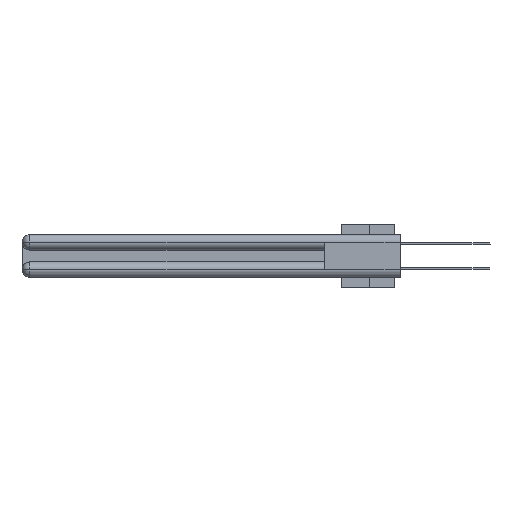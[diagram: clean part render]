
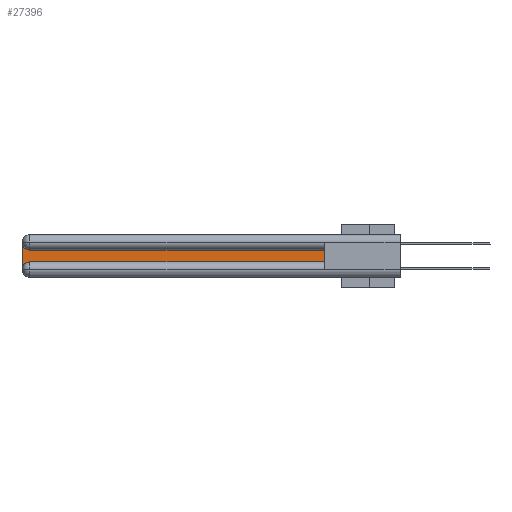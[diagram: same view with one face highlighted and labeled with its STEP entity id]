
A CAD part, left-side view. The second image highlights one B-rep face of the part: STEP entity #27396.
In plain terms, the highlighted planar face has unit normal (-1, 0, 0).
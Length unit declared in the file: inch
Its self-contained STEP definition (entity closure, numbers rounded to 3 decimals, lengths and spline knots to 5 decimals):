
#108 = VECTOR ( 'NONE', #23866, 39.37008 ) ;
#778 = CARTESIAN_POINT ( 'NONE',  ( 0.075, 3., -0.0625 ) ) ;
#1190 = CARTESIAN_POINT ( 'NONE',  ( 0.075, 2.94, -0.0625 ) ) ;
#3281 = CARTESIAN_POINT ( 'NONE',  ( 0.075, 0.6, -0.2175 ) ) ;
#3515 = LINE ( 'NONE', #32475, #12928 ) ;
#4697 = VERTEX_POINT ( 'NONE', #26727 ) ;
#5499 = AXIS2_PLACEMENT_3D ( 'NONE', #1190, #24079, #8109 ) ;
#5734 = VECTOR ( 'NONE', #16080, 39.37008 ) ;
#7492 = DIRECTION ( 'NONE',  ( 0., 0., -1. ) ) ;
#8109 = DIRECTION ( 'NONE',  ( 0., 0., -1. ) ) ;
#8886 = DIRECTION ( 'NONE',  ( 1., 0., 0. ) ) ;
#9432 = CARTESIAN_POINT ( 'NONE',  ( 0.075, 3., -0.2775 ) ) ;
#9581 = EDGE_LOOP ( 'NONE', ( #19163, #36787, #32205, #24450, #29224, #37832 ) ) ;
#10795 = CARTESIAN_POINT ( 'NONE',  ( 0.075, 2.94, -0.1225 ) ) ;
#12041 = DIRECTION ( 'NONE',  ( 1., 0., 0. ) ) ;
#12269 = EDGE_CURVE ( 'NONE', #4697, #40982, #3515, .T. ) ;
#12908 = VERTEX_POINT ( 'NONE', #10795 ) ;
#12928 = VECTOR ( 'NONE', #25778, 39.37008 ) ;
#13998 = CARTESIAN_POINT ( 'NONE',  ( 0.075, 3., -0.2175 ) ) ;
#15218 = CARTESIAN_POINT ( 'NONE',  ( 0.075, 0.6, -0.1225 ) ) ;
#15289 = EDGE_CURVE ( 'NONE', #38204, #4697, #19442, .T. ) ;
#16080 = DIRECTION ( 'NONE',  ( 0., -1., 0. ) ) ;
#16642 = EDGE_CURVE ( 'NONE', #40982, #12908, #36928, .T. ) ;
#17139 = LINE ( 'NONE', #13998, #108 ) ;
#17491 = EDGE_CURVE ( 'NONE', #22296, #38204, #28809, .T. ) ;
#17502 = DIRECTION ( 'NONE',  ( 0., 0., -1. ) ) ;
#18358 = CARTESIAN_POINT ( 'NONE',  ( 0.075, 2.94, -0.2175 ) ) ;
#19163 = ORIENTED_EDGE ( 'NONE', *, *, #16642, .T. ) ;
#19442 = LINE ( 'NONE', #3281, #5734 ) ;
#22052 = VECTOR ( 'NONE', #40298, 39.37008 ) ;
#22296 = VERTEX_POINT ( 'NONE', #9432 ) ;
#23500 = AXIS2_PLACEMENT_3D ( 'NONE', #36898, #8886, #7492 ) ;
#23866 = DIRECTION ( 'NONE',  ( 0., 0., -1. ) ) ;
#24079 = DIRECTION ( 'NONE',  ( 1., 0., 0. ) ) ;
#24450 = ORIENTED_EDGE ( 'NONE', *, *, #17491, .T. ) ;
#24831 = AXIS2_PLACEMENT_3D ( 'NONE', #30927, #12041, #17502 ) ;
#24955 = CARTESIAN_POINT ( 'NONE',  ( 0.075, 0.6, -0.1225 ) ) ;
#25778 = DIRECTION ( 'NONE',  ( 0., 0., 1. ) ) ;
#26727 = CARTESIAN_POINT ( 'NONE',  ( 0.075, 0.6, -0.2175 ) ) ;
#27242 = FACE_OUTER_BOUND ( 'NONE', #9581, .T. ) ;
#27396 = ADVANCED_FACE ( 'NONE', ( #27242 ), #33317, .F. ) ;
#28733 = EDGE_CURVE ( 'NONE', #33341, #22296, #17139, .T. ) ;
#28809 = CIRCLE ( 'NONE', #24831, 0.06 ) ;
#28889 = EDGE_CURVE ( 'NONE', #12908, #33341, #36320, .T. ) ;
#29224 = ORIENTED_EDGE ( 'NONE', *, *, #15289, .T. ) ;
#30927 = CARTESIAN_POINT ( 'NONE',  ( 0.075, 2.94, -0.2775 ) ) ;
#32205 = ORIENTED_EDGE ( 'NONE', *, *, #28733, .T. ) ;
#32475 = CARTESIAN_POINT ( 'NONE',  ( 0.075, 0.6, -0.2175 ) ) ;
#33317 = PLANE ( 'NONE',  #23500 ) ;
#33341 = VERTEX_POINT ( 'NONE', #778 ) ;
#36320 = CIRCLE ( 'NONE', #5499, 0.06 ) ;
#36787 = ORIENTED_EDGE ( 'NONE', *, *, #28889, .T. ) ;
#36898 = CARTESIAN_POINT ( 'NONE',  ( 0.075, 3., -0.1225 ) ) ;
#36928 = LINE ( 'NONE', #24955, #22052 ) ;
#37832 = ORIENTED_EDGE ( 'NONE', *, *, #12269, .T. ) ;
#38204 = VERTEX_POINT ( 'NONE', #18358 ) ;
#40298 = DIRECTION ( 'NONE',  ( 0., 1., 0. ) ) ;
#40982 = VERTEX_POINT ( 'NONE', #15218 ) ;
